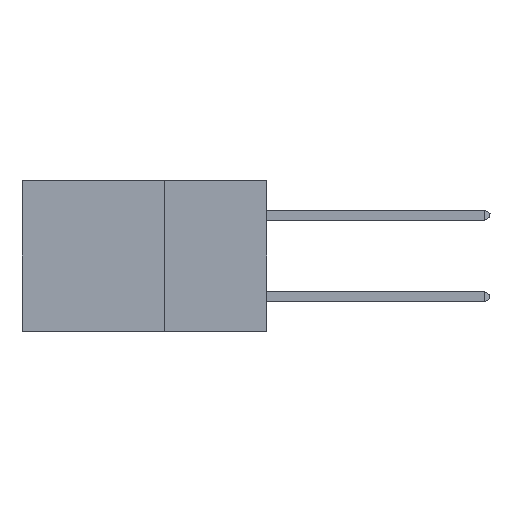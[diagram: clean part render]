
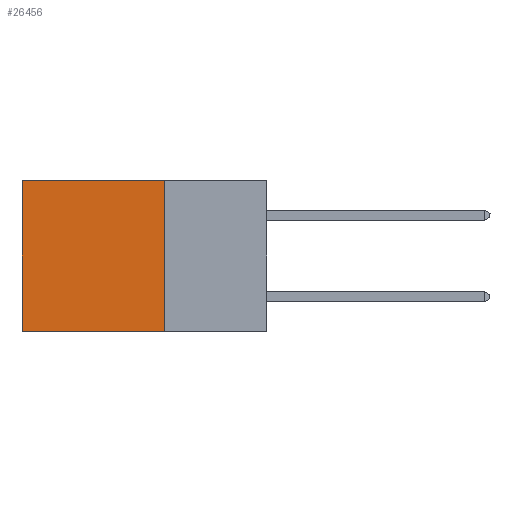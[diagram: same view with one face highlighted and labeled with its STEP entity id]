
A CAD part, left-side view. The second image highlights one B-rep face of the part: STEP entity #26456.
In plain terms, the highlighted planar face has unit normal (-1, 0, 0).
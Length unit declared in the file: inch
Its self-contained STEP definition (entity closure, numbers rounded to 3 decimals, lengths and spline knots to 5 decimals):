
#1037 = VECTOR ( 'NONE', #26410, 39.37008 ) ;
#1341 = ORIENTED_EDGE ( 'NONE', *, *, #33695, .T. ) ;
#2847 = EDGE_CURVE ( 'NONE', #36479, #17271, #12065, .T. ) ;
#4486 = DIRECTION ( 'NONE',  ( 0., 1., 0. ) ) ;
#4762 = LINE ( 'NONE', #7712, #17824 ) ;
#7712 = CARTESIAN_POINT ( 'NONE',  ( 0.2875, 0.25, -0.37 ) ) ;
#8907 = LINE ( 'NONE', #26837, #1037 ) ;
#8971 = VERTEX_POINT ( 'NONE', #27060 ) ;
#9182 = DIRECTION ( 'NONE',  ( 1., 0., 0. ) ) ;
#9310 = CARTESIAN_POINT ( 'NONE',  ( 0.2875, 0.25, 0. ) ) ;
#10936 = DIRECTION ( 'NONE',  ( 0., 0., -1. ) ) ;
#11534 = VECTOR ( 'NONE', #10936, 39.37008 ) ;
#11720 = EDGE_CURVE ( 'NONE', #17271, #20407, #4762, .T. ) ;
#12065 = LINE ( 'NONE', #43139, #29841 ) ;
#12099 = DIRECTION ( 'NONE',  ( 0., 0., -1. ) ) ;
#15877 = PLANE ( 'NONE',  #19896 ) ;
#17271 = VERTEX_POINT ( 'NONE', #36185 ) ;
#17824 = VECTOR ( 'NONE', #4486, 39.37008 ) ;
#19896 = AXIS2_PLACEMENT_3D ( 'NONE', #9310, #9182, #12099 ) ;
#20407 = VERTEX_POINT ( 'NONE', #39182 ) ;
#22130 = ORIENTED_EDGE ( 'NONE', *, *, #11720, .F. ) ;
#26410 = DIRECTION ( 'NONE',  ( 0., 1., 0. ) ) ;
#26456 = ADVANCED_FACE ( 'NONE', ( #40200 ), #15877, .F. ) ;
#26837 = CARTESIAN_POINT ( 'NONE',  ( 0.2875, 0.25, 0. ) ) ;
#27060 = CARTESIAN_POINT ( 'NONE',  ( 0.2875, 0.6, 0. ) ) ;
#29841 = VECTOR ( 'NONE', #36395, 39.37008 ) ;
#33695 = EDGE_CURVE ( 'NONE', #36479, #8971, #8907, .T. ) ;
#36085 = LINE ( 'NONE', #41175, #11534 ) ;
#36185 = CARTESIAN_POINT ( 'NONE',  ( 0.2875, 0.25, -0.37 ) ) ;
#36395 = DIRECTION ( 'NONE',  ( 0., 0., -1. ) ) ;
#36479 = VERTEX_POINT ( 'NONE', #40289 ) ;
#37325 = EDGE_CURVE ( 'NONE', #8971, #20407, #36085, .T. ) ;
#37439 = ORIENTED_EDGE ( 'NONE', *, *, #37325, .T. ) ;
#39182 = CARTESIAN_POINT ( 'NONE',  ( 0.2875, 0.6, -0.37 ) ) ;
#40200 = FACE_OUTER_BOUND ( 'NONE', #41383, .T. ) ;
#40289 = CARTESIAN_POINT ( 'NONE',  ( 0.2875, 0.25, 0. ) ) ;
#41175 = CARTESIAN_POINT ( 'NONE',  ( 0.2875, 0.6, 0. ) ) ;
#41383 = EDGE_LOOP ( 'NONE', ( #37439, #22130, #42017, #1341 ) ) ;
#42017 = ORIENTED_EDGE ( 'NONE', *, *, #2847, .F. ) ;
#43139 = CARTESIAN_POINT ( 'NONE',  ( 0.2875, 0.25, 0. ) ) ;
